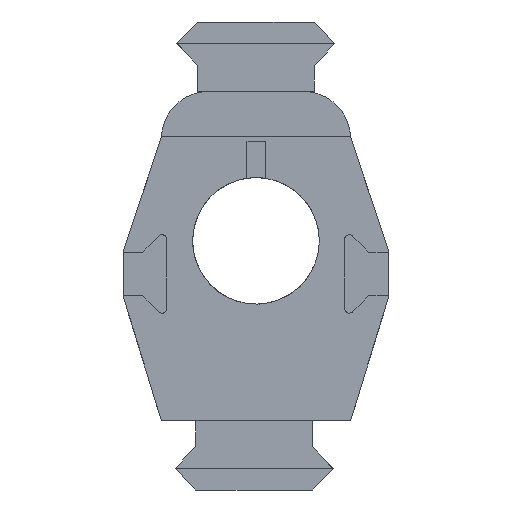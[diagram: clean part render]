
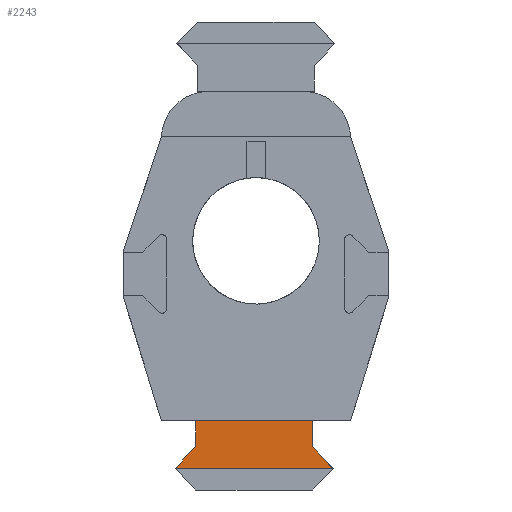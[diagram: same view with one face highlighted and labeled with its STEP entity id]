
A CAD part, front view. The second image highlights one B-rep face of the part: STEP entity #2243.
In plain terms, the highlighted planar face has unit normal (0, -1, 0).
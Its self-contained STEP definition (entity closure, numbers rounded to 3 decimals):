
#162=FACE_OUTER_BOUND('',#287,.T.);
#287=EDGE_LOOP('',(#1801,#1802,#1803,#1804,#1805,#1806));
#469=LINE('',#3479,#746);
#487=LINE('',#3514,#764);
#490=LINE('',#3520,#767);
#491=LINE('',#3523,#768);
#492=LINE('',#3525,#769);
#493=LINE('',#3526,#770);
#746=VECTOR('',#2821,10.);
#764=VECTOR('',#2841,10.);
#767=VECTOR('',#2846,10.);
#768=VECTOR('',#2849,10.);
#769=VECTOR('',#2850,10.);
#770=VECTOR('',#2851,10.);
#1012=VERTEX_POINT('',#3476);
#1013=VERTEX_POINT('',#3478);
#1029=VERTEX_POINT('',#3512);
#1031=VERTEX_POINT('',#3518);
#1032=VERTEX_POINT('',#3522);
#1033=VERTEX_POINT('',#3524);
#1281=EDGE_CURVE('',#1012,#1013,#469,.T.);
#1299=EDGE_CURVE('',#1029,#1012,#487,.T.);
#1302=EDGE_CURVE('',#1031,#1029,#490,.T.);
#1303=EDGE_CURVE('',#1032,#1031,#491,.T.);
#1304=EDGE_CURVE('',#1033,#1032,#492,.T.);
#1305=EDGE_CURVE('',#1013,#1033,#493,.T.);
#1801=ORIENTED_EDGE('',*,*,#1299,.F.);
#1802=ORIENTED_EDGE('',*,*,#1302,.F.);
#1803=ORIENTED_EDGE('',*,*,#1303,.F.);
#1804=ORIENTED_EDGE('',*,*,#1304,.F.);
#1805=ORIENTED_EDGE('',*,*,#1305,.F.);
#1806=ORIENTED_EDGE('',*,*,#1281,.F.);
#2122=PLANE('',#2425);
#2243=ADVANCED_FACE('',(#162),#2122,.F.);
#2425=AXIS2_PLACEMENT_3D('',#3521,#2847,#2848);
#2821=DIRECTION('',(0.691,0.,-0.723));
#2841=DIRECTION('',(0.,0.,-1.));
#2846=DIRECTION('',(1.,0.,0.));
#2847=DIRECTION('center_axis',(0.,1.,0.));
#2848=DIRECTION('ref_axis',(0.,0.,1.));
#2849=DIRECTION('',(0.,0.,1.));
#2850=DIRECTION('',(0.689,0.,0.725));
#2851=DIRECTION('',(-1.,0.,0.));
#3476=CARTESIAN_POINT('',(7.582,171.04,-16.235));
#3478=CARTESIAN_POINT('',(10.321,171.04,-19.102));
#3479=CARTESIAN_POINT('',(6.671,171.04,-15.282));
#3512=CARTESIAN_POINT('',(7.582,171.04,-12.7));
#3514=CARTESIAN_POINT('',(7.582,171.04,-19.129));
#3518=CARTESIAN_POINT('',(-8.09,171.04,-12.7));
#3520=CARTESIAN_POINT('',(-0.254,171.04,-12.7));
#3521=CARTESIAN_POINT('Origin',(-8.09,171.04,-22.022));
#3522=CARTESIAN_POINT('',(-8.09,171.04,-16.19));
#3523=CARTESIAN_POINT('',(-8.09,171.04,-17.361));
#3524=CARTESIAN_POINT('',(-10.858,171.04,-19.102));
#3525=CARTESIAN_POINT('',(-9.546,171.04,-17.721));
#3526=CARTESIAN_POINT('',(-8.09,171.04,-19.102));
